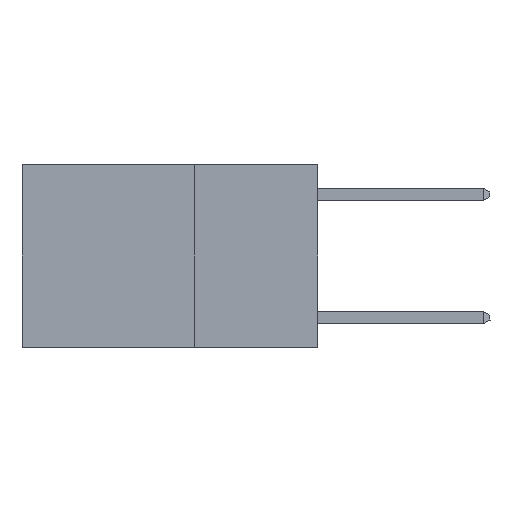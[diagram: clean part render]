
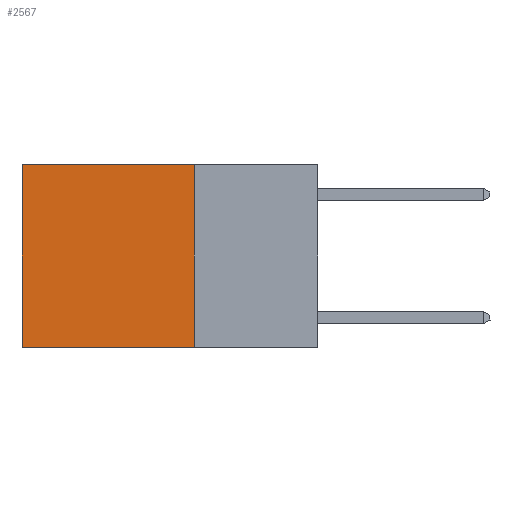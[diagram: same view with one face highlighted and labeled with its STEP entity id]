
A CAD part, left-side view. The second image highlights one B-rep face of the part: STEP entity #2567.
In plain terms, the highlighted planar face has unit normal (-1, 0, 0).
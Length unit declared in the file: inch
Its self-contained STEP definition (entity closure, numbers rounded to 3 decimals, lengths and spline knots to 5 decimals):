
#80 = ORIENTED_EDGE ( 'NONE', *, *, #4795, .F. ) ;
#448 = VECTOR ( 'NONE', #9719, 39.37008 ) ;
#2567 = ADVANCED_FACE ( 'NONE', ( #11464 ), #6396, .F. ) ;
#2659 = CARTESIAN_POINT ( 'NONE',  ( 0.2625, 0.25, -0.37 ) ) ;
#2877 = VECTOR ( 'NONE', #16297, 39.37008 ) ;
#3073 = CARTESIAN_POINT ( 'NONE',  ( 0.2625, 0.25, 0. ) ) ;
#3513 = ORIENTED_EDGE ( 'NONE', *, *, #10169, .T. ) ;
#4140 = DIRECTION ( 'NONE',  ( 0., 0., -1. ) ) ;
#4171 = VERTEX_POINT ( 'NONE', #16527 ) ;
#4392 = LINE ( 'NONE', #2659, #13899 ) ;
#4795 = EDGE_CURVE ( 'NONE', #4171, #14179, #6485, .T. ) ;
#6073 = EDGE_CURVE ( 'NONE', #14179, #11371, #4392, .T. ) ;
#6396 = PLANE ( 'NONE',  #8469 ) ;
#6485 = LINE ( 'NONE', #15044, #2877 ) ;
#6947 = VECTOR ( 'NONE', #4140, 39.37008 ) ;
#7537 = DIRECTION ( 'NONE',  ( 0., 0., -1. ) ) ;
#8177 = LINE ( 'NONE', #3073, #448 ) ;
#8469 = AXIS2_PLACEMENT_3D ( 'NONE', #10395, #9039, #7537 ) ;
#8996 = VERTEX_POINT ( 'NONE', #16553 ) ;
#9039 = DIRECTION ( 'NONE',  ( 1., 0., 0. ) ) ;
#9335 = DIRECTION ( 'NONE',  ( 0., 1., 0. ) ) ;
#9719 = DIRECTION ( 'NONE',  ( 0., 1., 0. ) ) ;
#10169 = EDGE_CURVE ( 'NONE', #8996, #11371, #10410, .T. ) ;
#10395 = CARTESIAN_POINT ( 'NONE',  ( 0.2625, 0.25, 0. ) ) ;
#10410 = LINE ( 'NONE', #10653, #6947 ) ;
#10653 = CARTESIAN_POINT ( 'NONE',  ( 0.2625, 0.6, 0. ) ) ;
#10928 = ORIENTED_EDGE ( 'NONE', *, *, #13764, .T. ) ;
#11371 = VERTEX_POINT ( 'NONE', #13806 ) ;
#11464 = FACE_OUTER_BOUND ( 'NONE', #12427, .T. ) ;
#12427 = EDGE_LOOP ( 'NONE', ( #3513, #13904, #80, #10928 ) ) ;
#13764 = EDGE_CURVE ( 'NONE', #4171, #8996, #8177, .T. ) ;
#13806 = CARTESIAN_POINT ( 'NONE',  ( 0.2625, 0.6, -0.37 ) ) ;
#13899 = VECTOR ( 'NONE', #9335, 39.37008 ) ;
#13904 = ORIENTED_EDGE ( 'NONE', *, *, #6073, .F. ) ;
#14179 = VERTEX_POINT ( 'NONE', #16626 ) ;
#15044 = CARTESIAN_POINT ( 'NONE',  ( 0.2625, 0.25, 0. ) ) ;
#16297 = DIRECTION ( 'NONE',  ( 0., 0., -1. ) ) ;
#16527 = CARTESIAN_POINT ( 'NONE',  ( 0.2625, 0.25, 0. ) ) ;
#16553 = CARTESIAN_POINT ( 'NONE',  ( 0.2625, 0.6, 0. ) ) ;
#16626 = CARTESIAN_POINT ( 'NONE',  ( 0.2625, 0.25, -0.37 ) ) ;
